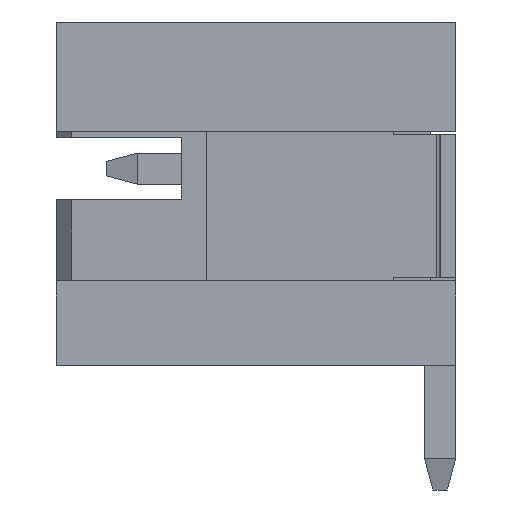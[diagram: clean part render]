
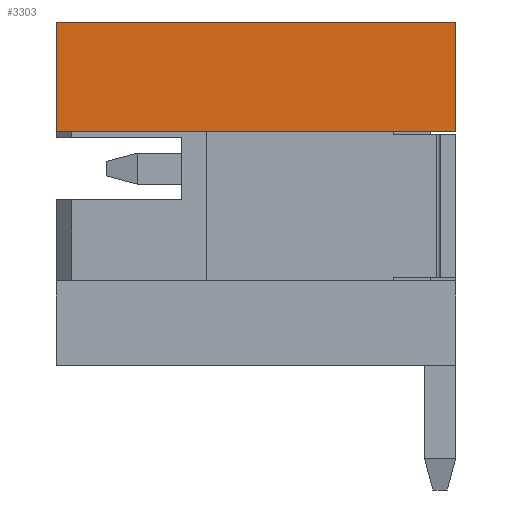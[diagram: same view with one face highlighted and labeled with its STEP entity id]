
A CAD part, left-side view. The second image highlights one B-rep face of the part: STEP entity #3303.
In plain terms, the highlighted planar face has unit normal (-1, 0, 0).
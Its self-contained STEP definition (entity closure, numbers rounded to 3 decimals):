
#99 = EDGE_CURVE ( 'NONE', #8820, #5601, #8036, .T. ) ;
#935 = ORIENTED_EDGE ( 'NONE', *, *, #10122, .F. ) ;
#1001 = VERTEX_POINT ( 'NONE', #2083 ) ;
#1094 = VECTOR ( 'NONE', #1409, 1000. ) ;
#1409 = DIRECTION ( 'NONE',  ( 0., 1., 0. ) ) ;
#1648 = CARTESIAN_POINT ( 'NONE',  ( -3., 0., 0.6 ) ) ;
#2083 = CARTESIAN_POINT ( 'NONE',  ( -3., 6.4, 2.35 ) ) ;
#2945 = CARTESIAN_POINT ( 'NONE',  ( -3., 6.4, 2.35 ) ) ;
#3047 = LINE ( 'NONE', #6005, #6297 ) ;
#3303 = ADVANCED_FACE ( 'NONE', ( #7353 ), #3527, .F. ) ;
#3527 = PLANE ( 'NONE',  #4183 ) ;
#3605 = DIRECTION ( 'NONE',  ( 0., 0., -1. ) ) ;
#3873 = ORIENTED_EDGE ( 'NONE', *, *, #99, .F. ) ;
#4056 = VECTOR ( 'NONE', #8585, 1000. ) ;
#4183 = AXIS2_PLACEMENT_3D ( 'NONE', #4472, #11061, #3605 ) ;
#4472 = CARTESIAN_POINT ( 'NONE',  ( -3., 0., 0. ) ) ;
#4525 = ORIENTED_EDGE ( 'NONE', *, *, #8281, .F. ) ;
#5020 = EDGE_CURVE ( 'NONE', #5601, #1001, #3047, .T. ) ;
#5601 = VERTEX_POINT ( 'NONE', #6803 ) ;
#6005 = CARTESIAN_POINT ( 'NONE',  ( -3., 6.4, 2.35 ) ) ;
#6285 = CARTESIAN_POINT ( 'NONE',  ( -3., 0., 2.35 ) ) ;
#6297 = VECTOR ( 'NONE', #10806, 1000. ) ;
#6803 = CARTESIAN_POINT ( 'NONE',  ( -3., 6.4, 0.6 ) ) ;
#7284 = LINE ( 'NONE', #2945, #4056 ) ;
#7353 = FACE_OUTER_BOUND ( 'NONE', #11507, .T. ) ;
#7696 = VECTOR ( 'NONE', #8187, 1000. ) ;
#8036 = LINE ( 'NONE', #8981, #1094 ) ;
#8187 = DIRECTION ( 'NONE',  ( 0., 0., -1. ) ) ;
#8281 = EDGE_CURVE ( 'NONE', #1001, #9491, #7284, .T. ) ;
#8585 = DIRECTION ( 'NONE',  ( 0., -1., 0. ) ) ;
#8820 = VERTEX_POINT ( 'NONE', #1648 ) ;
#8981 = CARTESIAN_POINT ( 'NONE',  ( -3., 0., 0.6 ) ) ;
#9217 = CARTESIAN_POINT ( 'NONE',  ( -3., 0., 2.35 ) ) ;
#9491 = VERTEX_POINT ( 'NONE', #9217 ) ;
#10122 = EDGE_CURVE ( 'NONE', #9491, #8820, #10637, .T. ) ;
#10637 = LINE ( 'NONE', #6285, #7696 ) ;
#10806 = DIRECTION ( 'NONE',  ( 0., 0., 1. ) ) ;
#11061 = DIRECTION ( 'NONE',  ( 1., 0., 0. ) ) ;
#11507 = EDGE_LOOP ( 'NONE', ( #11519, #3873, #935, #4525 ) ) ;
#11519 = ORIENTED_EDGE ( 'NONE', *, *, #5020, .F. ) ;
